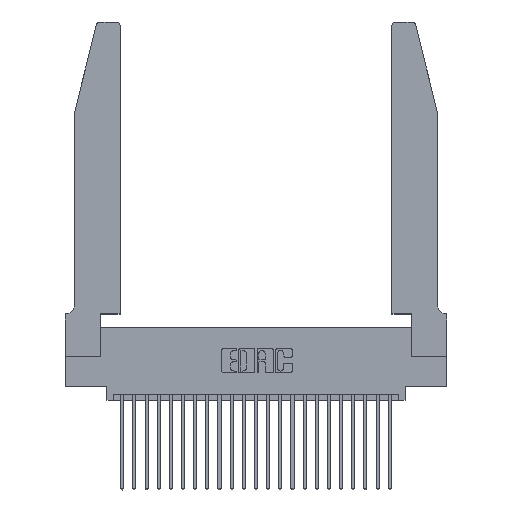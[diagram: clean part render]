
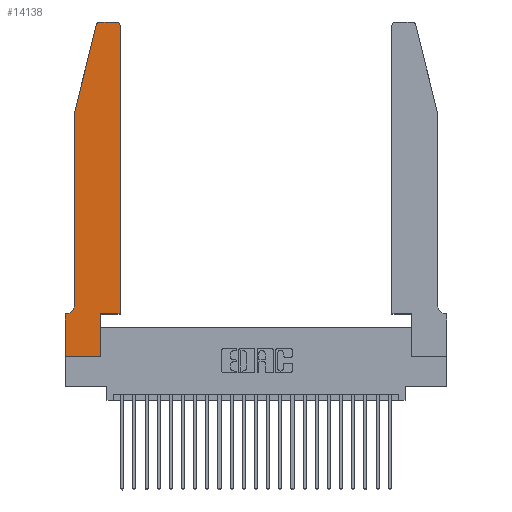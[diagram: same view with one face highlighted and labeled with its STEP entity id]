
A CAD part, top view. The second image highlights one B-rep face of the part: STEP entity #14138.
In plain terms, the highlighted planar face has unit normal (0, 0, 1).
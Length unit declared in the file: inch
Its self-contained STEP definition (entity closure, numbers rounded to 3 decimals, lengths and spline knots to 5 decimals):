
#6 = EDGE_CURVE ( 'NONE', #4814, #7982, #151, .T. ) ;
#151 = LINE ( 'NONE', #14994, #11349 ) ;
#825 = VERTEX_POINT ( 'NONE', #24319 ) ;
#1371 = AXIS2_PLACEMENT_3D ( 'NONE', #16455, #20212, #14183 ) ;
#1580 = ORIENTED_EDGE ( 'NONE', *, *, #17877, .T. ) ;
#1676 = EDGE_CURVE ( 'NONE', #15977, #4814, #23285, .T. ) ;
#1875 = CARTESIAN_POINT ( 'NONE',  ( 0.0055, 0.42, 0.37 ) ) ;
#1930 = ORIENTED_EDGE ( 'NONE', *, *, #9600, .T. ) ;
#2388 = CIRCLE ( 'NONE', #1371, 0.03 ) ;
#2459 = LINE ( 'NONE', #19291, #24328 ) ;
#2949 = VERTEX_POINT ( 'NONE', #15269 ) ;
#3280 = AXIS2_PLACEMENT_3D ( 'NONE', #4254, #12381, #15115 ) ;
#3620 = ORIENTED_EDGE ( 'NONE', *, *, #4701, .T. ) ;
#3684 = CARTESIAN_POINT ( 'NONE',  ( 0.4505, 0.35, 0.37 ) ) ;
#3959 = ORIENTED_EDGE ( 'NONE', *, *, #17711, .T. ) ;
#4254 = CARTESIAN_POINT ( 'NONE',  ( 0., 0.35, 0.37 ) ) ;
#4701 = EDGE_CURVE ( 'NONE', #2949, #17062, #2459, .T. ) ;
#4789 = LINE ( 'NONE', #19263, #12519 ) ;
#4814 = VERTEX_POINT ( 'NONE', #3684 ) ;
#4908 = DIRECTION ( 'NONE',  ( 0., 0., 1. ) ) ;
#4984 = CARTESIAN_POINT ( 'NONE',  ( 0.4505, 0.35, 0.37 ) ) ;
#5011 = VERTEX_POINT ( 'NONE', #12182 ) ;
#5125 = CARTESIAN_POINT ( 'NONE',  ( 0.2605, 2.75, 0.37 ) ) ;
#6167 = CIRCLE ( 'NONE', #10578, 0.03 ) ;
#6199 = ORIENTED_EDGE ( 'NONE', *, *, #13482, .T. ) ;
#6221 = DIRECTION ( 'NONE',  ( 0., 0., -1. ) ) ;
#7021 = DIRECTION ( 'NONE',  ( 1., 0., 0. ) ) ;
#7316 = CARTESIAN_POINT ( 'NONE',  ( 0.0055, 0.35, 0.37 ) ) ;
#7566 = ORIENTED_EDGE ( 'NONE', *, *, #1676, .T. ) ;
#7796 = DIRECTION ( 'NONE',  ( -1., 0., 0. ) ) ;
#7982 = VERTEX_POINT ( 'NONE', #21992 ) ;
#8353 = CARTESIAN_POINT ( 'NONE',  ( 0.0755, 2., 0.37 ) ) ;
#8584 = LINE ( 'NONE', #11656, #13186 ) ;
#9451 = ORIENTED_EDGE ( 'NONE', *, *, #24673, .T. ) ;
#9600 = EDGE_CURVE ( 'NONE', #23496, #825, #4789, .T. ) ;
#10033 = EDGE_CURVE ( 'NONE', #825, #23838, #14952, .T. ) ;
#10133 = CARTESIAN_POINT ( 'NONE',  ( 0., 0., 0.37 ) ) ;
#10578 = AXIS2_PLACEMENT_3D ( 'NONE', #18782, #4908, #20482 ) ;
#11266 = VECTOR ( 'NONE', #21196, 39.37008 ) ;
#11289 = CARTESIAN_POINT ( 'NONE',  ( 0.2865, 0.35, 0.37 ) ) ;
#11349 = VECTOR ( 'NONE', #19620, 39.37008 ) ;
#11640 = VECTOR ( 'NONE', #7021, 39.37008 ) ;
#11656 = CARTESIAN_POINT ( 'NONE',  ( 0., 0., 0.37 ) ) ;
#11678 = CARTESIAN_POINT ( 'NONE',  ( 0.2865, 0.35, 0.37 ) ) ;
#11743 = VECTOR ( 'NONE', #13590, 39.37008 ) ;
#11859 = EDGE_CURVE ( 'NONE', #5011, #15977, #21616, .T. ) ;
#12182 = CARTESIAN_POINT ( 'NONE',  ( 0.2865, 0., 0.37 ) ) ;
#12306 = FACE_OUTER_BOUND ( 'NONE', #22004, .T. ) ;
#12381 = DIRECTION ( 'NONE',  ( 0., 0., 1. ) ) ;
#12519 = VECTOR ( 'NONE', #19092, 39.37008 ) ;
#13186 = VECTOR ( 'NONE', #13622, 39.37008 ) ;
#13365 = ORIENTED_EDGE ( 'NONE', *, *, #10033, .T. ) ;
#13482 = EDGE_CURVE ( 'NONE', #22409, #14588, #6167, .T. ) ;
#13590 = DIRECTION ( 'NONE',  ( -0.239, -0.971, 0. ) ) ;
#13622 = DIRECTION ( 'NONE',  ( 1., 0., 0. ) ) ;
#13872 = DIRECTION ( 'NONE',  ( 0., 1., 0. ) ) ;
#14138 = ADVANCED_FACE ( 'NONE', ( #12306 ), #18675, .T. ) ;
#14183 = DIRECTION ( 'NONE',  ( 1., 0., 0. ) ) ;
#14588 = VERTEX_POINT ( 'NONE', #21772 ) ;
#14856 = ORIENTED_EDGE ( 'NONE', *, *, #19566, .T. ) ;
#14952 = CIRCLE ( 'NONE', #23316, 0.07 ) ;
#14994 = CARTESIAN_POINT ( 'NONE',  ( 0.4505, 0.35, 0.37 ) ) ;
#15115 = DIRECTION ( 'NONE',  ( 1., 0., 0. ) ) ;
#15269 = CARTESIAN_POINT ( 'NONE',  ( 0., 0.35, 0.37 ) ) ;
#15499 = CARTESIAN_POINT ( 'NONE',  ( 0.0755, 2., 0.37 ) ) ;
#15977 = VERTEX_POINT ( 'NONE', #11289 ) ;
#16452 = VECTOR ( 'NONE', #13872, 39.37008 ) ;
#16455 = CARTESIAN_POINT ( 'NONE',  ( 0.4205, 2.72, 0.37 ) ) ;
#16460 = VECTOR ( 'NONE', #17247, 39.37008 ) ;
#16656 = CARTESIAN_POINT ( 'NONE',  ( 0.284, 2.75, 0.37 ) ) ;
#16830 = CARTESIAN_POINT ( 'NONE',  ( 0.4205, 2.75, 0.37 ) ) ;
#17062 = VERTEX_POINT ( 'NONE', #10133 ) ;
#17247 = DIRECTION ( 'NONE',  ( -1., 0., 0. ) ) ;
#17711 = EDGE_CURVE ( 'NONE', #24370, #22409, #20154, .T. ) ;
#17877 = EDGE_CURVE ( 'NONE', #23838, #2949, #22238, .T. ) ;
#18675 = PLANE ( 'NONE',  #3280 ) ;
#18782 = CARTESIAN_POINT ( 'NONE',  ( 0.284, 2.72, 0.37 ) ) ;
#19092 = DIRECTION ( 'NONE',  ( 0., -1., 0. ) ) ;
#19263 = CARTESIAN_POINT ( 'NONE',  ( 0.0755, 2., 0.37 ) ) ;
#19291 = CARTESIAN_POINT ( 'NONE',  ( 0., 0., 0.37 ) ) ;
#19421 = LINE ( 'NONE', #15499, #11743 ) ;
#19566 = EDGE_CURVE ( 'NONE', #14588, #23496, #19421, .T. ) ;
#19620 = DIRECTION ( 'NONE',  ( 0., 1., 0. ) ) ;
#20154 = LINE ( 'NONE', #5125, #11266 ) ;
#20212 = DIRECTION ( 'NONE',  ( 0., 0., 1. ) ) ;
#20317 = ORIENTED_EDGE ( 'NONE', *, *, #11859, .T. ) ;
#20482 = DIRECTION ( 'NONE',  ( 1., 0., 0. ) ) ;
#21032 = EDGE_CURVE ( 'NONE', #7982, #24370, #2388, .T. ) ;
#21196 = DIRECTION ( 'NONE',  ( -1., 0., 0. ) ) ;
#21228 = ORIENTED_EDGE ( 'NONE', *, *, #6, .T. ) ;
#21616 = LINE ( 'NONE', #11678, #16452 ) ;
#21772 = CARTESIAN_POINT ( 'NONE',  ( 0.25487, 2.72718, 0.37 ) ) ;
#21992 = CARTESIAN_POINT ( 'NONE',  ( 0.4505, 2.72, 0.37 ) ) ;
#22004 = EDGE_LOOP ( 'NONE', ( #3959, #6199, #14856, #1930, #13365, #1580, #3620, #9451, #20317, #7566, #21228, #23370 ) ) ;
#22238 = LINE ( 'NONE', #25008, #16460 ) ;
#22409 = VERTEX_POINT ( 'NONE', #16656 ) ;
#23285 = LINE ( 'NONE', #4984, #11640 ) ;
#23290 = DIRECTION ( 'NONE',  ( 0., -1., 0. ) ) ;
#23316 = AXIS2_PLACEMENT_3D ( 'NONE', #1875, #6221, #7796 ) ;
#23370 = ORIENTED_EDGE ( 'NONE', *, *, #21032, .T. ) ;
#23496 = VERTEX_POINT ( 'NONE', #8353 ) ;
#23838 = VERTEX_POINT ( 'NONE', #7316 ) ;
#24319 = CARTESIAN_POINT ( 'NONE',  ( 0.0755, 0.42, 0.37 ) ) ;
#24328 = VECTOR ( 'NONE', #23290, 39.37008 ) ;
#24370 = VERTEX_POINT ( 'NONE', #16830 ) ;
#24673 = EDGE_CURVE ( 'NONE', #17062, #5011, #8584, .T. ) ;
#25008 = CARTESIAN_POINT ( 'NONE',  ( 0.0755, 0.35, 0.37 ) ) ;
